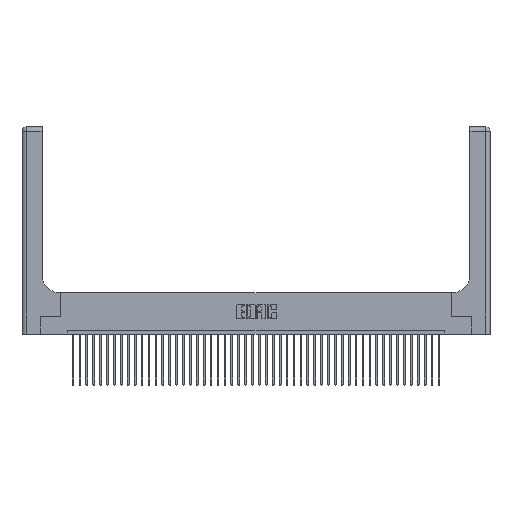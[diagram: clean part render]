
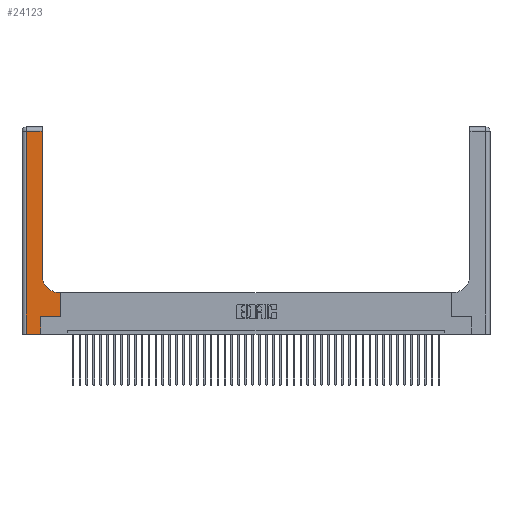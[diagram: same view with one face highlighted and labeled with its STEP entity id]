
A CAD part, top view. The second image highlights one B-rep face of the part: STEP entity #24123.
In plain terms, the highlighted planar face has unit normal (0, 0, 1).
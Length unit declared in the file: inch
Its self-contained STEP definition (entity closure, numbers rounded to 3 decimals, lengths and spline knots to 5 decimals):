
#1287 = LINE ( 'NONE', #17558, #24274 ) ;
#1502 = DIRECTION ( 'NONE',  ( 1., 0., 0. ) ) ;
#1820 = EDGE_CURVE ( 'NONE', #40987, #10974, #10154, .T. ) ;
#2093 = AXIS2_PLACEMENT_3D ( 'NONE', #38035, #21299, #8231 ) ;
#2765 = LINE ( 'NONE', #37693, #31596 ) ;
#3248 = CARTESIAN_POINT ( 'NONE',  ( 0.2915, 0.85, 0.37 ) ) ;
#3360 = ORIENTED_EDGE ( 'NONE', *, *, #9874, .T. ) ;
#5107 = EDGE_CURVE ( 'NONE', #33969, #27428, #9382, .T. ) ;
#5212 = CARTESIAN_POINT ( 'NONE',  ( 0., 3., 0.37 ) ) ;
#6541 = CARTESIAN_POINT ( 'NONE',  ( 0.2915, 2.94, 0.37 ) ) ;
#6656 = EDGE_CURVE ( 'NONE', #31358, #21720, #37285, .T. ) ;
#6885 = FACE_OUTER_BOUND ( 'NONE', #13096, .T. ) ;
#8231 = DIRECTION ( 'NONE',  ( 1., 0., 0. ) ) ;
#8574 = VERTEX_POINT ( 'NONE', #28335 ) ;
#9382 = LINE ( 'NONE', #41250, #35628 ) ;
#9418 = EDGE_CURVE ( 'NONE', #8574, #31358, #2765, .T. ) ;
#9874 = EDGE_CURVE ( 'NONE', #43188, #31436, #28945, .T. ) ;
#10154 = LINE ( 'NONE', #41883, #41145 ) ;
#10839 = DIRECTION ( 'NONE',  ( 1., 0., 0. ) ) ;
#10974 = VERTEX_POINT ( 'NONE', #6541 ) ;
#12623 = ORIENTED_EDGE ( 'NONE', *, *, #1820, .T. ) ;
#12953 = CARTESIAN_POINT ( 'NONE',  ( 0.269, 0.25, 0.37 ) ) ;
#13096 = EDGE_LOOP ( 'NONE', ( #12623, #29860, #3360, #23528, #20853, #33852, #21129, #28061, #40584 ) ) ;
#13751 = EDGE_CURVE ( 'NONE', #21720, #33969, #1287, .T. ) ;
#14436 = DIRECTION ( 'NONE',  ( 0., 1., 0. ) ) ;
#15944 = EDGE_CURVE ( 'NONE', #31436, #8574, #17640, .T. ) ;
#16267 = DIRECTION ( 'NONE',  ( 0., -1., 0. ) ) ;
#16624 = VECTOR ( 'NONE', #10839, 39.37008 ) ;
#17558 = CARTESIAN_POINT ( 'NONE',  ( 0.5585, 0.25, 0.37 ) ) ;
#17640 = LINE ( 'NONE', #41473, #16624 ) ;
#18907 = PLANE ( 'NONE',  #24492 ) ;
#19037 = CARTESIAN_POINT ( 'NONE',  ( 0.5585, 0.25, 0.37 ) ) ;
#20066 = DIRECTION ( 'NONE',  ( 0., 1., 0. ) ) ;
#20790 = DIRECTION ( 'NONE',  ( -1., 0., 0. ) ) ;
#20853 = ORIENTED_EDGE ( 'NONE', *, *, #9418, .T. ) ;
#21129 = ORIENTED_EDGE ( 'NONE', *, *, #13751, .T. ) ;
#21299 = DIRECTION ( 'NONE',  ( 0., 0., -1. ) ) ;
#21720 = VERTEX_POINT ( 'NONE', #19037 ) ;
#21791 = CARTESIAN_POINT ( 'NONE',  ( 0.5585, 0.6, 0.37 ) ) ;
#23528 = ORIENTED_EDGE ( 'NONE', *, *, #15944, .T. ) ;
#23782 = VECTOR ( 'NONE', #33324, 39.37008 ) ;
#24123 = ADVANCED_FACE ( 'NONE', ( #6885 ), #18907, .F. ) ;
#24274 = VECTOR ( 'NONE', #14436, 39.37008 ) ;
#24492 = AXIS2_PLACEMENT_3D ( 'NONE', #5212, #25811, #25342 ) ;
#25342 = DIRECTION ( 'NONE',  ( -1., 0., 0. ) ) ;
#25811 = DIRECTION ( 'NONE',  ( 0., 0., -1. ) ) ;
#27428 = VERTEX_POINT ( 'NONE', #33181 ) ;
#28061 = ORIENTED_EDGE ( 'NONE', *, *, #5107, .T. ) ;
#28335 = CARTESIAN_POINT ( 'NONE',  ( 0.269, 0., 0.37 ) ) ;
#28945 = LINE ( 'NONE', #40041, #35890 ) ;
#29374 = CARTESIAN_POINT ( 'NONE',  ( 0.269, 0.25, 0.37 ) ) ;
#29860 = ORIENTED_EDGE ( 'NONE', *, *, #31500, .T. ) ;
#31358 = VERTEX_POINT ( 'NONE', #12953 ) ;
#31436 = VERTEX_POINT ( 'NONE', #33632 ) ;
#31500 = EDGE_CURVE ( 'NONE', #10974, #43188, #35552, .T. ) ;
#31596 = VECTOR ( 'NONE', #20066, 39.37008 ) ;
#31719 = EDGE_CURVE ( 'NONE', #27428, #40987, #33973, .T. ) ;
#31782 = DIRECTION ( 'NONE',  ( 0., 1., 0. ) ) ;
#33181 = CARTESIAN_POINT ( 'NONE',  ( 0.5415, 0.6, 0.37 ) ) ;
#33324 = DIRECTION ( 'NONE',  ( -1., 0., 0. ) ) ;
#33632 = CARTESIAN_POINT ( 'NONE',  ( 0.06, 0., 0.37 ) ) ;
#33852 = ORIENTED_EDGE ( 'NONE', *, *, #6656, .T. ) ;
#33969 = VERTEX_POINT ( 'NONE', #21791 ) ;
#33973 = CIRCLE ( 'NONE', #2093, 0.25 ) ;
#35181 = CARTESIAN_POINT ( 'NONE',  ( 0.06, 2.94, 0.37 ) ) ;
#35552 = LINE ( 'NONE', #41903, #23782 ) ;
#35628 = VECTOR ( 'NONE', #20790, 39.37008 ) ;
#35890 = VECTOR ( 'NONE', #16267, 39.37008 ) ;
#36728 = VECTOR ( 'NONE', #1502, 39.37008 ) ;
#37285 = LINE ( 'NONE', #29374, #36728 ) ;
#37693 = CARTESIAN_POINT ( 'NONE',  ( 0.269, 0., 0.37 ) ) ;
#38035 = CARTESIAN_POINT ( 'NONE',  ( 0.5415, 0.85, 0.37 ) ) ;
#40041 = CARTESIAN_POINT ( 'NONE',  ( 0.06, 3., 0.37 ) ) ;
#40584 = ORIENTED_EDGE ( 'NONE', *, *, #31719, .T. ) ;
#40987 = VERTEX_POINT ( 'NONE', #3248 ) ;
#41145 = VECTOR ( 'NONE', #31782, 39.37008 ) ;
#41250 = CARTESIAN_POINT ( 'NONE',  ( 0.2915, 0.6, 0.37 ) ) ;
#41473 = CARTESIAN_POINT ( 'NONE',  ( 0., 0., 0.37 ) ) ;
#41883 = CARTESIAN_POINT ( 'NONE',  ( 0.2915, 3., 0.37 ) ) ;
#41903 = CARTESIAN_POINT ( 'NONE',  ( 0., 2.94, 0.37 ) ) ;
#43188 = VERTEX_POINT ( 'NONE', #35181 ) ;
